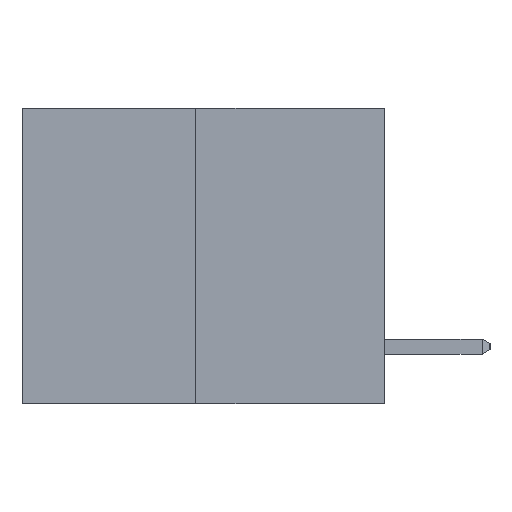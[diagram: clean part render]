
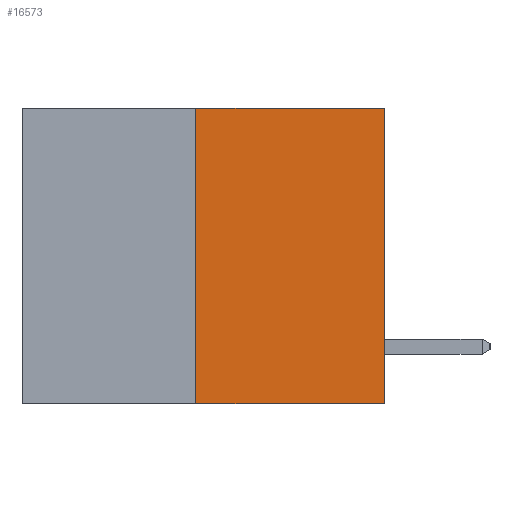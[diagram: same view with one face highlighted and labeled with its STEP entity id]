
A CAD part, left-side view. The second image highlights one B-rep face of the part: STEP entity #16573.
In plain terms, the highlighted planar face has unit normal (-1, 0, 0).
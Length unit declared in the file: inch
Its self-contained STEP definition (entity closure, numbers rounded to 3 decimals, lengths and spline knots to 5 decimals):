
#570 = VECTOR ( 'NONE', #3273, 39.37008 ) ;
#729 = VECTOR ( 'NONE', #11155, 39.37008 ) ;
#963 = AXIS2_PLACEMENT_3D ( 'NONE', #13098, #1249, #6514 ) ;
#1249 = DIRECTION ( 'NONE',  ( 1., 0., 0. ) ) ;
#1729 = CARTESIAN_POINT ( 'NONE',  ( 0., 0.6, -0.49 ) ) ;
#2051 = CARTESIAN_POINT ( 'NONE',  ( 0., 0.6, 0. ) ) ;
#2642 = VERTEX_POINT ( 'NONE', #12766 ) ;
#3083 = CARTESIAN_POINT ( 'NONE',  ( 0., 0., 0. ) ) ;
#3273 = DIRECTION ( 'NONE',  ( 0., -1., 0. ) ) ;
#3584 = LINE ( 'NONE', #8700, #729 ) ;
#3608 = DIRECTION ( 'NONE',  ( 0., 0., 1. ) ) ;
#3880 = EDGE_LOOP ( 'NONE', ( #15928, #11927, #9740, #12968 ) ) ;
#3929 = VECTOR ( 'NONE', #3608, 39.37008 ) ;
#4269 = DIRECTION ( 'NONE',  ( 0., -1., 0. ) ) ;
#4413 = LINE ( 'NONE', #1729, #11490 ) ;
#4414 = FACE_OUTER_BOUND ( 'NONE', #3880, .T. ) ;
#5512 = VERTEX_POINT ( 'NONE', #9791 ) ;
#6514 = DIRECTION ( 'NONE',  ( 0., 0., -1. ) ) ;
#8700 = CARTESIAN_POINT ( 'NONE',  ( 0., 0., 0. ) ) ;
#9698 = EDGE_CURVE ( 'NONE', #13304, #12171, #3584, .T. ) ;
#9740 = ORIENTED_EDGE ( 'NONE', *, *, #9698, .T. ) ;
#9791 = CARTESIAN_POINT ( 'NONE',  ( 0., 0.312, 0. ) ) ;
#10507 = PLANE ( 'NONE',  #963 ) ;
#11112 = EDGE_CURVE ( 'NONE', #2642, #5512, #13616, .T. ) ;
#11155 = DIRECTION ( 'NONE',  ( 0., 0., 1. ) ) ;
#11217 = CARTESIAN_POINT ( 'NONE',  ( 0., 0.312, -0.49 ) ) ;
#11490 = VECTOR ( 'NONE', #4269, 39.37008 ) ;
#11927 = ORIENTED_EDGE ( 'NONE', *, *, #15649, .T. ) ;
#12171 = VERTEX_POINT ( 'NONE', #3083 ) ;
#12400 = CARTESIAN_POINT ( 'NONE',  ( 0., 0., -0.49 ) ) ;
#12512 = LINE ( 'NONE', #2051, #570 ) ;
#12766 = CARTESIAN_POINT ( 'NONE',  ( 0., 0.312, -0.49 ) ) ;
#12968 = ORIENTED_EDGE ( 'NONE', *, *, #16281, .F. ) ;
#13098 = CARTESIAN_POINT ( 'NONE',  ( 0., 0.6, 0. ) ) ;
#13304 = VERTEX_POINT ( 'NONE', #12400 ) ;
#13616 = LINE ( 'NONE', #11217, #3929 ) ;
#15649 = EDGE_CURVE ( 'NONE', #2642, #13304, #4413, .T. ) ;
#15928 = ORIENTED_EDGE ( 'NONE', *, *, #11112, .F. ) ;
#16281 = EDGE_CURVE ( 'NONE', #5512, #12171, #12512, .T. ) ;
#16573 = ADVANCED_FACE ( 'NONE', ( #4414 ), #10507, .F. ) ;
